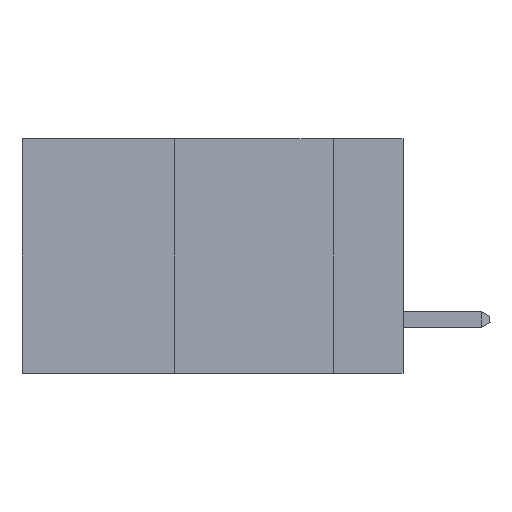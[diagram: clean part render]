
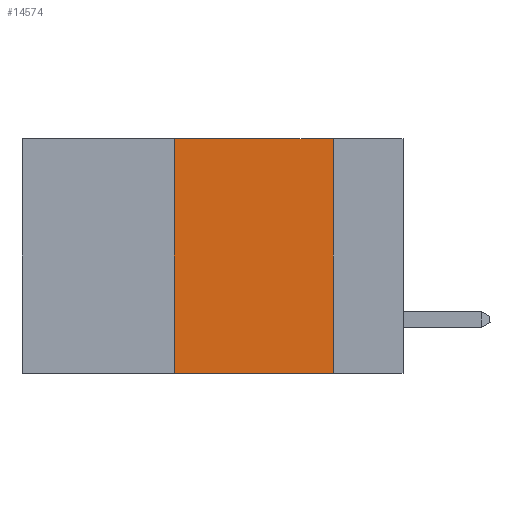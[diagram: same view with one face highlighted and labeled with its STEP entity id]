
A CAD part, left-side view. The second image highlights one B-rep face of the part: STEP entity #14574.
In plain terms, the highlighted planar face has unit normal (-1, 0, 0).
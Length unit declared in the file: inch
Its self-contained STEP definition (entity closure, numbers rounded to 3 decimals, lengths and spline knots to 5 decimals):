
#349 = AXIS2_PLACEMENT_3D ( 'NONE', #2924, #1679, #8588 ) ;
#581 = VECTOR ( 'NONE', #10709, 39.37008 ) ;
#1099 = VERTEX_POINT ( 'NONE', #6169 ) ;
#1336 = EDGE_LOOP ( 'NONE', ( #9705, #10309, #10549, #9483 ) ) ;
#1528 = DIRECTION ( 'NONE',  ( 0., 0., -1. ) ) ;
#1679 = DIRECTION ( 'NONE',  ( 1., 0., 0. ) ) ;
#1852 = LINE ( 'NONE', #9548, #581 ) ;
#2468 = VECTOR ( 'NONE', #12595, 39.37008 ) ;
#2869 = CARTESIAN_POINT ( 'NONE',  ( 0., 0.11, 0. ) ) ;
#2924 = CARTESIAN_POINT ( 'NONE',  ( 0., 0.6, 0. ) ) ;
#4729 = EDGE_CURVE ( 'NONE', #1099, #9333, #8455, .T. ) ;
#5633 = EDGE_CURVE ( 'NONE', #13643, #5877, #9728, .T. ) ;
#5877 = VERTEX_POINT ( 'NONE', #5958 ) ;
#5958 = CARTESIAN_POINT ( 'NONE',  ( 0., 0.11, -0.37 ) ) ;
#6169 = CARTESIAN_POINT ( 'NONE',  ( 0., 0.36, -0.37 ) ) ;
#6281 = CARTESIAN_POINT ( 'NONE',  ( 0., 0.36, 0. ) ) ;
#6627 = CARTESIAN_POINT ( 'NONE',  ( 0., 0.11, 0. ) ) ;
#8455 = LINE ( 'NONE', #6281, #11556 ) ;
#8588 = DIRECTION ( 'NONE',  ( 0., 0., -1. ) ) ;
#8692 = PLANE ( 'NONE',  #349 ) ;
#9333 = VERTEX_POINT ( 'NONE', #11839 ) ;
#9370 = EDGE_CURVE ( 'NONE', #1099, #5877, #1852, .T. ) ;
#9483 = ORIENTED_EDGE ( 'NONE', *, *, #9370, .T. ) ;
#9548 = CARTESIAN_POINT ( 'NONE',  ( 0., 0.6, -0.37 ) ) ;
#9705 = ORIENTED_EDGE ( 'NONE', *, *, #5633, .F. ) ;
#9728 = LINE ( 'NONE', #2869, #12461 ) ;
#10309 = ORIENTED_EDGE ( 'NONE', *, *, #12307, .F. ) ;
#10549 = ORIENTED_EDGE ( 'NONE', *, *, #4729, .F. ) ;
#10709 = DIRECTION ( 'NONE',  ( 0., -1., 0. ) ) ;
#11556 = VECTOR ( 'NONE', #12852, 39.37008 ) ;
#11839 = CARTESIAN_POINT ( 'NONE',  ( 0., 0.36, 0. ) ) ;
#12209 = FACE_OUTER_BOUND ( 'NONE', #1336, .T. ) ;
#12307 = EDGE_CURVE ( 'NONE', #9333, #13643, #14850, .T. ) ;
#12461 = VECTOR ( 'NONE', #1528, 39.37008 ) ;
#12595 = DIRECTION ( 'NONE',  ( 0., -1., 0. ) ) ;
#12852 = DIRECTION ( 'NONE',  ( 0., 0., 1. ) ) ;
#13643 = VERTEX_POINT ( 'NONE', #6627 ) ;
#14574 = ADVANCED_FACE ( 'NONE', ( #12209 ), #8692, .F. ) ;
#14850 = LINE ( 'NONE', #14940, #2468 ) ;
#14940 = CARTESIAN_POINT ( 'NONE',  ( 0., 0.6, 0. ) ) ;
